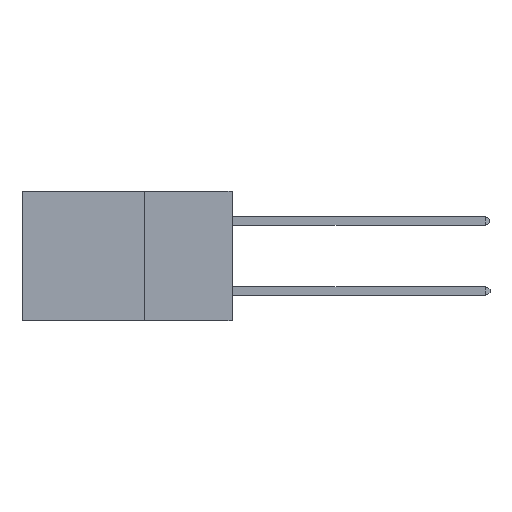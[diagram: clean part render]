
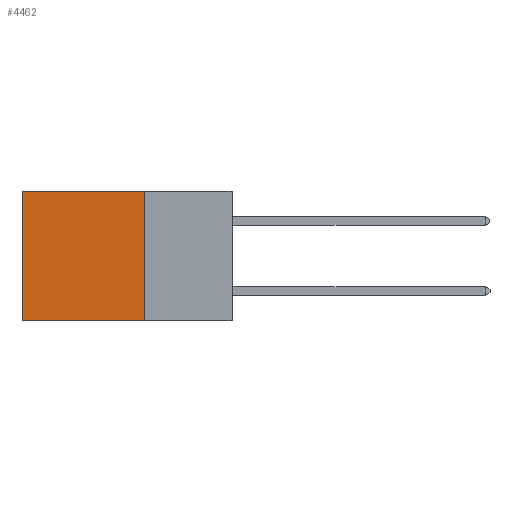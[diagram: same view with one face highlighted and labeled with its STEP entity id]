
A CAD part, left-side view. The second image highlights one B-rep face of the part: STEP entity #4462.
In plain terms, the highlighted planar face has unit normal (-1, 0, 0).
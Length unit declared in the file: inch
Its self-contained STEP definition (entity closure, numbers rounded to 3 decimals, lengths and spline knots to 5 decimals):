
#282 = EDGE_CURVE ( 'NONE', #18296, #17029, #2763, .T. ) ;
#865 = ORIENTED_EDGE ( 'NONE', *, *, #10509, .T. ) ;
#954 = CARTESIAN_POINT ( 'NONE',  ( 0.2875, 0.25, 0. ) ) ;
#993 = CARTESIAN_POINT ( 'NONE',  ( 0.2875, 0.25, 0. ) ) ;
#1193 = CARTESIAN_POINT ( 'NONE',  ( 0.2875, 0.25, -0.37 ) ) ;
#1981 = DIRECTION ( 'NONE',  ( 0., 1., 0. ) ) ;
#2673 = DIRECTION ( 'NONE',  ( 0., 0., -1. ) ) ;
#2763 = LINE ( 'NONE', #3064, #15509 ) ;
#2953 = VECTOR ( 'NONE', #1981, 39.37008 ) ;
#3064 = CARTESIAN_POINT ( 'NONE',  ( 0.2875, 0.25, 0. ) ) ;
#4462 = ADVANCED_FACE ( 'NONE', ( #9998 ), #17576, .F. ) ;
#4618 = DIRECTION ( 'NONE',  ( 0., 1., 0. ) ) ;
#7185 = EDGE_LOOP ( 'NONE', ( #15690, #12491, #8185, #865 ) ) ;
#8185 = ORIENTED_EDGE ( 'NONE', *, *, #282, .F. ) ;
#9710 = AXIS2_PLACEMENT_3D ( 'NONE', #954, #12518, #2673 ) ;
#9998 = FACE_OUTER_BOUND ( 'NONE', #7185, .T. ) ;
#10509 = EDGE_CURVE ( 'NONE', #18296, #14086, #15701, .T. ) ;
#11805 = CARTESIAN_POINT ( 'NONE',  ( 0.2875, 0.25, 0. ) ) ;
#11829 = CARTESIAN_POINT ( 'NONE',  ( 0.2875, 0.6, -0.37 ) ) ;
#12096 = DIRECTION ( 'NONE',  ( 0., 0., -1. ) ) ;
#12491 = ORIENTED_EDGE ( 'NONE', *, *, #14941, .F. ) ;
#12518 = DIRECTION ( 'NONE',  ( 1., 0., 0. ) ) ;
#13581 = LINE ( 'NONE', #13753, #17582 ) ;
#13753 = CARTESIAN_POINT ( 'NONE',  ( 0.2875, 0.6, 0. ) ) ;
#13991 = VECTOR ( 'NONE', #4618, 39.37008 ) ;
#14086 = VERTEX_POINT ( 'NONE', #18075 ) ;
#14552 = CARTESIAN_POINT ( 'NONE',  ( 0.2875, 0.25, -0.37 ) ) ;
#14941 = EDGE_CURVE ( 'NONE', #17029, #16643, #18444, .T. ) ;
#15509 = VECTOR ( 'NONE', #19160, 39.37008 ) ;
#15690 = ORIENTED_EDGE ( 'NONE', *, *, #18127, .T. ) ;
#15701 = LINE ( 'NONE', #11805, #2953 ) ;
#16643 = VERTEX_POINT ( 'NONE', #11829 ) ;
#17029 = VERTEX_POINT ( 'NONE', #1193 ) ;
#17576 = PLANE ( 'NONE',  #9710 ) ;
#17582 = VECTOR ( 'NONE', #12096, 39.37008 ) ;
#18075 = CARTESIAN_POINT ( 'NONE',  ( 0.2875, 0.6, 0. ) ) ;
#18127 = EDGE_CURVE ( 'NONE', #14086, #16643, #13581, .T. ) ;
#18296 = VERTEX_POINT ( 'NONE', #993 ) ;
#18444 = LINE ( 'NONE', #14552, #13991 ) ;
#19160 = DIRECTION ( 'NONE',  ( 0., 0., -1. ) ) ;
